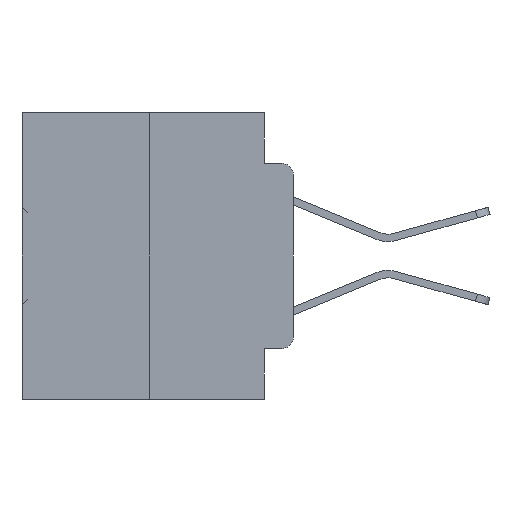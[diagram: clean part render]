
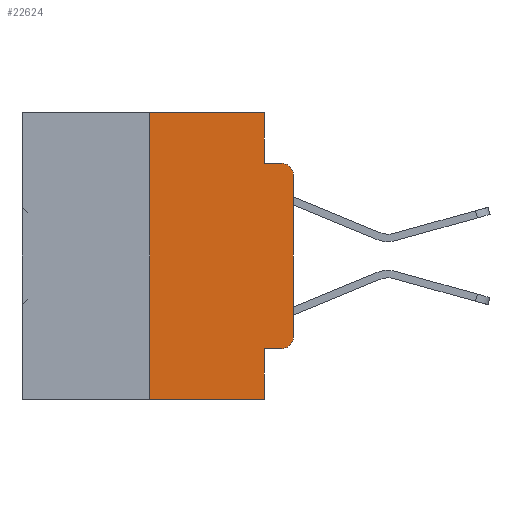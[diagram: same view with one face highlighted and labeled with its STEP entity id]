
A CAD part, left-side view. The second image highlights one B-rep face of the part: STEP entity #22624.
In plain terms, the highlighted planar face has unit normal (-1, 0, 0).
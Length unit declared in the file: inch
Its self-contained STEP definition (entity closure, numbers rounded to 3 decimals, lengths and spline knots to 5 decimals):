
#235 = LINE ( 'NONE', #14047, #21289 ) ;
#240 = EDGE_CURVE ( 'NONE', #19427, #1618, #29929, .T. ) ;
#477 = DIRECTION ( 'NONE',  ( 1., 0., 0. ) ) ;
#790 = DIRECTION ( 'NONE',  ( -1., 0., 0. ) ) ;
#1246 = VECTOR ( 'NONE', #2099, 39.37008 ) ;
#1373 = CARTESIAN_POINT ( 'NONE',  ( 0., 0.051, 0. ) ) ;
#1411 = ORIENTED_EDGE ( 'NONE', *, *, #7742, .T. ) ;
#1618 = VERTEX_POINT ( 'NONE', #13233 ) ;
#1649 = VECTOR ( 'NONE', #22099, 39.37008 ) ;
#1732 = CARTESIAN_POINT ( 'NONE',  ( 0., 0.051, -0.4115 ) ) ;
#2099 = DIRECTION ( 'NONE',  ( 0., -1., 0. ) ) ;
#2958 = DIRECTION ( 'NONE',  ( 0., 0., 1. ) ) ;
#2967 = ORIENTED_EDGE ( 'NONE', *, *, #16794, .T. ) ;
#2973 = CIRCLE ( 'NONE', #16274, 0.02 ) ;
#4079 = EDGE_LOOP ( 'NONE', ( #1411, #2967, #11944, #22141, #10674, #17587, #28377, #13662, #15987, #27095 ) ) ;
#4538 = CIRCLE ( 'NONE', #20876, 0.02 ) ;
#4579 = LINE ( 'NONE', #1732, #11106 ) ;
#5537 = LINE ( 'NONE', #20110, #9669 ) ;
#6549 = LINE ( 'NONE', #11842, #19317 ) ;
#6580 = CARTESIAN_POINT ( 'NONE',  ( 0., 0.051, 0. ) ) ;
#7742 = EDGE_CURVE ( 'NONE', #20330, #21951, #235, .T. ) ;
#7883 = CARTESIAN_POINT ( 'NONE',  ( 0., 0.051, 0. ) ) ;
#8263 = LINE ( 'NONE', #22848, #27703 ) ;
#8989 = FACE_OUTER_BOUND ( 'NONE', #4079, .T. ) ;
#9669 = VECTOR ( 'NONE', #11957, 39.37008 ) ;
#10674 = ORIENTED_EDGE ( 'NONE', *, *, #20680, .F. ) ;
#11106 = VECTOR ( 'NONE', #33588, 39.37008 ) ;
#11819 = VERTEX_POINT ( 'NONE', #25316 ) ;
#11842 = CARTESIAN_POINT ( 'NONE',  ( 0., 0.25, 0. ) ) ;
#11944 = ORIENTED_EDGE ( 'NONE', *, *, #36801, .F. ) ;
#11957 = DIRECTION ( 'NONE',  ( 0., -1., 0. ) ) ;
#12182 = VERTEX_POINT ( 'NONE', #29896 ) ;
#12573 = VERTEX_POINT ( 'NONE', #17883 ) ;
#12959 = CARTESIAN_POINT ( 'NONE',  ( 0., 0.02, -0.3915 ) ) ;
#13210 = EDGE_CURVE ( 'NONE', #12182, #24396, #4579, .T. ) ;
#13233 = CARTESIAN_POINT ( 'NONE',  ( 0., 0.051, -0.0885 ) ) ;
#13662 = ORIENTED_EDGE ( 'NONE', *, *, #20456, .F. ) ;
#13788 = CARTESIAN_POINT ( 'NONE',  ( 0., 0.051, -0.5 ) ) ;
#14047 = CARTESIAN_POINT ( 'NONE',  ( 0., 0., 0. ) ) ;
#14244 = DIRECTION ( 'NONE',  ( 0., 0., 1. ) ) ;
#14464 = EDGE_CURVE ( 'NONE', #12573, #11819, #6549, .T. ) ;
#15987 = ORIENTED_EDGE ( 'NONE', *, *, #13210, .T. ) ;
#16274 = AXIS2_PLACEMENT_3D ( 'NONE', #26761, #790, #32650 ) ;
#16794 = EDGE_CURVE ( 'NONE', #21951, #29911, #2973, .T. ) ;
#17587 = ORIENTED_EDGE ( 'NONE', *, *, #14464, .F. ) ;
#17883 = CARTESIAN_POINT ( 'NONE',  ( 0., 0.25, -0.5 ) ) ;
#18143 = DIRECTION ( 'NONE',  ( 0., 0., -1. ) ) ;
#18469 = VECTOR ( 'NONE', #18143, 39.37008 ) ;
#19317 = VECTOR ( 'NONE', #2958, 39.37008 ) ;
#19427 = VERTEX_POINT ( 'NONE', #1373 ) ;
#20110 = CARTESIAN_POINT ( 'NONE',  ( 0., 0.473, -0.5 ) ) ;
#20330 = VERTEX_POINT ( 'NONE', #30319 ) ;
#20456 = EDGE_CURVE ( 'NONE', #12182, #28696, #21916, .T. ) ;
#20680 = EDGE_CURVE ( 'NONE', #11819, #19427, #8263, .T. ) ;
#20737 = DIRECTION ( 'NONE',  ( 0., 0., -1. ) ) ;
#20876 = AXIS2_PLACEMENT_3D ( 'NONE', #12959, #30622, #21858 ) ;
#20912 = AXIS2_PLACEMENT_3D ( 'NONE', #32157, #477, #20737 ) ;
#21289 = VECTOR ( 'NONE', #14244, 39.37008 ) ;
#21858 = DIRECTION ( 'NONE',  ( 0., 0., -1. ) ) ;
#21916 = LINE ( 'NONE', #7883, #1649 ) ;
#21951 = VERTEX_POINT ( 'NONE', #36770 ) ;
#22099 = DIRECTION ( 'NONE',  ( 0., 0., -1. ) ) ;
#22141 = ORIENTED_EDGE ( 'NONE', *, *, #240, .F. ) ;
#22624 = ADVANCED_FACE ( 'NONE', ( #8989 ), #35364, .F. ) ;
#22848 = CARTESIAN_POINT ( 'NONE',  ( 0., 0.473, 0. ) ) ;
#24080 = EDGE_CURVE ( 'NONE', #24396, #20330, #4538, .T. ) ;
#24307 = CARTESIAN_POINT ( 'NONE',  ( 0., 0.02, -0.0885 ) ) ;
#24396 = VERTEX_POINT ( 'NONE', #36637 ) ;
#25024 = LINE ( 'NONE', #33210, #1246 ) ;
#25316 = CARTESIAN_POINT ( 'NONE',  ( 0., 0.25, 0. ) ) ;
#26761 = CARTESIAN_POINT ( 'NONE',  ( 0., 0.02, -0.1085 ) ) ;
#27095 = ORIENTED_EDGE ( 'NONE', *, *, #24080, .T. ) ;
#27703 = VECTOR ( 'NONE', #31611, 39.37008 ) ;
#28377 = ORIENTED_EDGE ( 'NONE', *, *, #29623, .T. ) ;
#28696 = VERTEX_POINT ( 'NONE', #13788 ) ;
#29623 = EDGE_CURVE ( 'NONE', #12573, #28696, #5537, .T. ) ;
#29896 = CARTESIAN_POINT ( 'NONE',  ( 0., 0.051, -0.4115 ) ) ;
#29911 = VERTEX_POINT ( 'NONE', #24307 ) ;
#29929 = LINE ( 'NONE', #6580, #18469 ) ;
#30319 = CARTESIAN_POINT ( 'NONE',  ( 0., 0., -0.3915 ) ) ;
#30622 = DIRECTION ( 'NONE',  ( -1., 0., 0. ) ) ;
#31611 = DIRECTION ( 'NONE',  ( 0., -1., 0. ) ) ;
#32157 = CARTESIAN_POINT ( 'NONE',  ( 0., 0.473, 0. ) ) ;
#32650 = DIRECTION ( 'NONE',  ( 0., 0., -1. ) ) ;
#33210 = CARTESIAN_POINT ( 'NONE',  ( 0., 0.051, -0.0885 ) ) ;
#33588 = DIRECTION ( 'NONE',  ( 0., -1., 0. ) ) ;
#35364 = PLANE ( 'NONE',  #20912 ) ;
#36637 = CARTESIAN_POINT ( 'NONE',  ( 0., 0.02, -0.4115 ) ) ;
#36770 = CARTESIAN_POINT ( 'NONE',  ( 0., 0., -0.1085 ) ) ;
#36801 = EDGE_CURVE ( 'NONE', #1618, #29911, #25024, .T. ) ;
